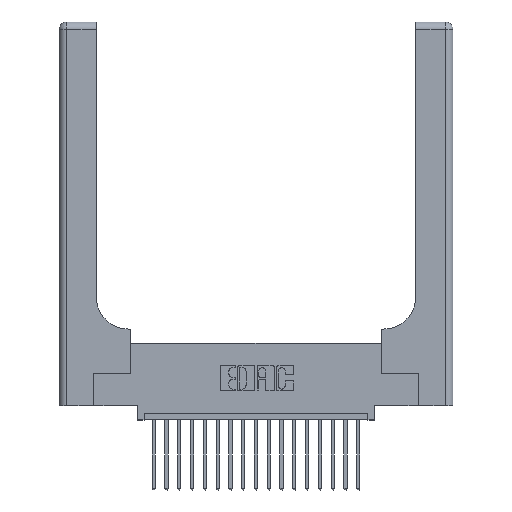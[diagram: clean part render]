
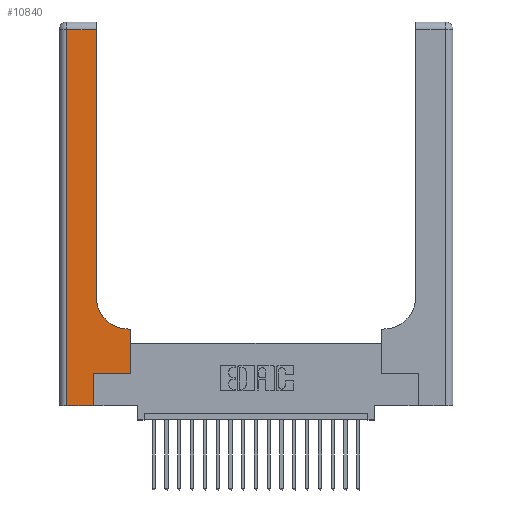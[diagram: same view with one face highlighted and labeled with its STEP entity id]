
A CAD part, top view. The second image highlights one B-rep face of the part: STEP entity #10840.
In plain terms, the highlighted planar face has unit normal (0, 0, 1).
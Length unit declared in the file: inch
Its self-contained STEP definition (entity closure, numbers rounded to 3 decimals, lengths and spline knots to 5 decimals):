
#629 = DIRECTION ( 'NONE',  ( 0., 1., 0. ) ) ;
#882 = LINE ( 'NONE', #5786, #8671 ) ;
#935 = VERTEX_POINT ( 'NONE', #10032 ) ;
#1022 = DIRECTION ( 'NONE',  ( -1., 0., 0. ) ) ;
#1096 = VERTEX_POINT ( 'NONE', #11928 ) ;
#1266 = EDGE_CURVE ( 'NONE', #8186, #3796, #18731, .T. ) ;
#2034 = ORIENTED_EDGE ( 'NONE', *, *, #4197, .T. ) ;
#2198 = CARTESIAN_POINT ( 'NONE',  ( 0.5585, 0.25, 0.37 ) ) ;
#2653 = FACE_OUTER_BOUND ( 'NONE', #2912, .T. ) ;
#2912 = EDGE_LOOP ( 'NONE', ( #4444, #2034, #18866, #19070, #16688, #14671, #5578, #17856, #6011 ) ) ;
#3256 = EDGE_CURVE ( 'NONE', #15446, #8186, #16360, .T. ) ;
#3796 = VERTEX_POINT ( 'NONE', #10806 ) ;
#4192 = DIRECTION ( 'NONE',  ( 1., 0., 0. ) ) ;
#4197 = EDGE_CURVE ( 'NONE', #1096, #17415, #20527, .T. ) ;
#4277 = DIRECTION ( 'NONE',  ( -1., 0., 0. ) ) ;
#4438 = VECTOR ( 'NONE', #4488, 39.37008 ) ;
#4444 = ORIENTED_EDGE ( 'NONE', *, *, #4966, .T. ) ;
#4488 = DIRECTION ( 'NONE',  ( 1., 0., 0. ) ) ;
#4680 = VERTEX_POINT ( 'NONE', #6874 ) ;
#4966 = EDGE_CURVE ( 'NONE', #935, #1096, #10961, .T. ) ;
#5211 = VECTOR ( 'NONE', #13361, 39.37008 ) ;
#5440 = DIRECTION ( 'NONE',  ( 1., 0., 0. ) ) ;
#5578 = ORIENTED_EDGE ( 'NONE', *, *, #3256, .T. ) ;
#5786 = CARTESIAN_POINT ( 'NONE',  ( 0.269, 0.25, 0.37 ) ) ;
#5888 = DIRECTION ( 'NONE',  ( -1., 0., 0. ) ) ;
#6011 = ORIENTED_EDGE ( 'NONE', *, *, #13907, .T. ) ;
#6451 = EDGE_CURVE ( 'NONE', #17415, #9542, #14518, .T. ) ;
#6874 = CARTESIAN_POINT ( 'NONE',  ( 0.269, 0.25, 0.37 ) ) ;
#7297 = VERTEX_POINT ( 'NONE', #14707 ) ;
#7318 = CARTESIAN_POINT ( 'NONE',  ( 0.06, 3., 0.37 ) ) ;
#7513 = PLANE ( 'NONE',  #9763 ) ;
#7791 = LINE ( 'NONE', #11383, #5211 ) ;
#8186 = VERTEX_POINT ( 'NONE', #11090 ) ;
#8490 = CARTESIAN_POINT ( 'NONE',  ( 0.06, 2.94, 0.37 ) ) ;
#8671 = VECTOR ( 'NONE', #4192, 39.37008 ) ;
#9040 = CIRCLE ( 'NONE', #14964, 0.25 ) ;
#9197 = DIRECTION ( 'NONE',  ( 0., -1., 0. ) ) ;
#9214 = CARTESIAN_POINT ( 'NONE',  ( 0.2915, 0.6, 0.37 ) ) ;
#9304 = DIRECTION ( 'NONE',  ( 0., 0., -1. ) ) ;
#9542 = VERTEX_POINT ( 'NONE', #21177 ) ;
#9763 = AXIS2_PLACEMENT_3D ( 'NONE', #12534, #9304, #5888 ) ;
#10032 = CARTESIAN_POINT ( 'NONE',  ( 0.2915, 0.85, 0.37 ) ) ;
#10380 = VECTOR ( 'NONE', #629, 39.37008 ) ;
#10611 = CARTESIAN_POINT ( 'NONE',  ( 0.5415, 0.85, 0.37 ) ) ;
#10777 = EDGE_CURVE ( 'NONE', #4680, #15446, #882, .T. ) ;
#10806 = CARTESIAN_POINT ( 'NONE',  ( 0.5415, 0.6, 0.37 ) ) ;
#10840 = ADVANCED_FACE ( 'NONE', ( #2653 ), #7513, .F. ) ;
#10897 = CARTESIAN_POINT ( 'NONE',  ( 0., 2.94, 0.37 ) ) ;
#10915 = DIRECTION ( 'NONE',  ( 0., 1., 0. ) ) ;
#10961 = LINE ( 'NONE', #20741, #12551 ) ;
#11090 = CARTESIAN_POINT ( 'NONE',  ( 0.5585, 0.6, 0.37 ) ) ;
#11383 = CARTESIAN_POINT ( 'NONE',  ( 0.269, 0., 0.37 ) ) ;
#11928 = CARTESIAN_POINT ( 'NONE',  ( 0.2915, 2.94, 0.37 ) ) ;
#12534 = CARTESIAN_POINT ( 'NONE',  ( 0., 3., 0.37 ) ) ;
#12551 = VECTOR ( 'NONE', #10915, 39.37008 ) ;
#12576 = CARTESIAN_POINT ( 'NONE',  ( 0.5585, 0.25, 0.37 ) ) ;
#13361 = DIRECTION ( 'NONE',  ( 0., 1., 0. ) ) ;
#13907 = EDGE_CURVE ( 'NONE', #3796, #935, #9040, .T. ) ;
#14518 = LINE ( 'NONE', #7318, #21233 ) ;
#14671 = ORIENTED_EDGE ( 'NONE', *, *, #10777, .T. ) ;
#14707 = CARTESIAN_POINT ( 'NONE',  ( 0.269, 0., 0.37 ) ) ;
#14964 = AXIS2_PLACEMENT_3D ( 'NONE', #10611, #15420, #5440 ) ;
#15420 = DIRECTION ( 'NONE',  ( 0., 0., -1. ) ) ;
#15446 = VERTEX_POINT ( 'NONE', #12576 ) ;
#16360 = LINE ( 'NONE', #2198, #10380 ) ;
#16686 = LINE ( 'NONE', #19505, #4438 ) ;
#16688 = ORIENTED_EDGE ( 'NONE', *, *, #20030, .T. ) ;
#17205 = VECTOR ( 'NONE', #1022, 39.37008 ) ;
#17415 = VERTEX_POINT ( 'NONE', #8490 ) ;
#17856 = ORIENTED_EDGE ( 'NONE', *, *, #1266, .T. ) ;
#18731 = LINE ( 'NONE', #9214, #21313 ) ;
#18866 = ORIENTED_EDGE ( 'NONE', *, *, #6451, .T. ) ;
#19070 = ORIENTED_EDGE ( 'NONE', *, *, #19341, .T. ) ;
#19341 = EDGE_CURVE ( 'NONE', #9542, #7297, #16686, .T. ) ;
#19505 = CARTESIAN_POINT ( 'NONE',  ( 0., 0., 0.37 ) ) ;
#20030 = EDGE_CURVE ( 'NONE', #7297, #4680, #7791, .T. ) ;
#20527 = LINE ( 'NONE', #10897, #17205 ) ;
#20741 = CARTESIAN_POINT ( 'NONE',  ( 0.2915, 3., 0.37 ) ) ;
#21177 = CARTESIAN_POINT ( 'NONE',  ( 0.06, 0., 0.37 ) ) ;
#21233 = VECTOR ( 'NONE', #9197, 39.37008 ) ;
#21313 = VECTOR ( 'NONE', #4277, 39.37008 ) ;
